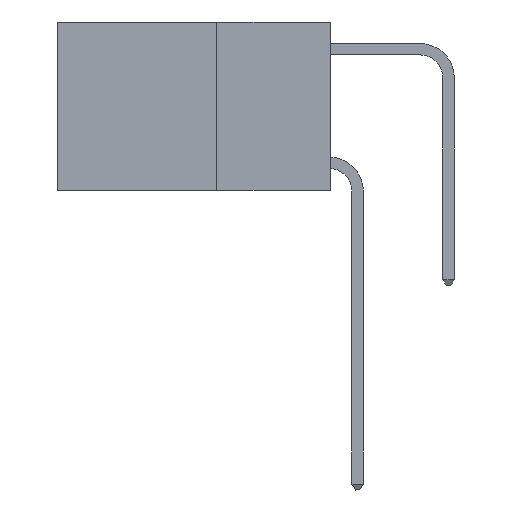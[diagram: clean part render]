
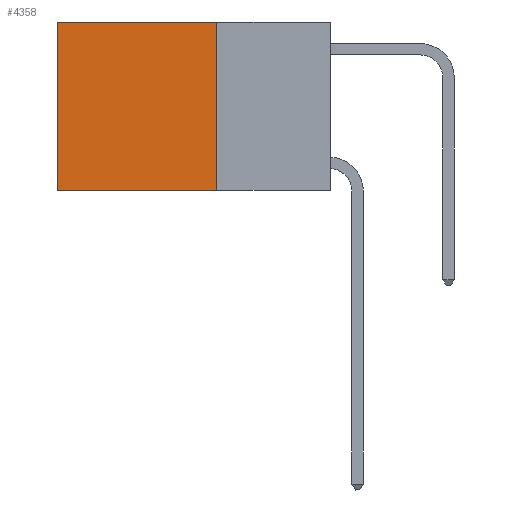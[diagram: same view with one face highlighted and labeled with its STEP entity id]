
A CAD part, left-side view. The second image highlights one B-rep face of the part: STEP entity #4358.
In plain terms, the highlighted planar face has unit normal (-1, 0, 0).
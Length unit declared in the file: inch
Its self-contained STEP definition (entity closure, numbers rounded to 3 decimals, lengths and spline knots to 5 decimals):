
#334 = EDGE_CURVE ( 'NONE', #12512, #3990, #8209, .T. ) ;
#675 = VECTOR ( 'NONE', #4784, 39.37008 ) ;
#962 = VERTEX_POINT ( 'NONE', #2156 ) ;
#1251 = EDGE_CURVE ( 'NONE', #7937, #962, #14690, .T. ) ;
#1430 = CARTESIAN_POINT ( 'NONE',  ( 0.2625, 0.25, 0. ) ) ;
#1451 = VECTOR ( 'NONE', #10331, 39.37008 ) ;
#1916 = CARTESIAN_POINT ( 'NONE',  ( 0.2625, 0.25, -0.37 ) ) ;
#2156 = CARTESIAN_POINT ( 'NONE',  ( 0.2625, 0.6, 0. ) ) ;
#3990 = VERTEX_POINT ( 'NONE', #4826 ) ;
#4358 = ADVANCED_FACE ( 'NONE', ( #16212 ), #9805, .F. ) ;
#4748 = EDGE_CURVE ( 'NONE', #7937, #12512, #12236, .T. ) ;
#4784 = DIRECTION ( 'NONE',  ( 0., 0., -1. ) ) ;
#4826 = CARTESIAN_POINT ( 'NONE',  ( 0.2625, 0.6, -0.37 ) ) ;
#5518 = DIRECTION ( 'NONE',  ( 0., 1., 0. ) ) ;
#6842 = EDGE_LOOP ( 'NONE', ( #9349, #10776, #9980, #16669 ) ) ;
#7898 = VECTOR ( 'NONE', #8095, 39.37008 ) ;
#7937 = VERTEX_POINT ( 'NONE', #1430 ) ;
#8095 = DIRECTION ( 'NONE',  ( 0., 1., 0. ) ) ;
#8209 = LINE ( 'NONE', #1916, #11579 ) ;
#8336 = AXIS2_PLACEMENT_3D ( 'NONE', #8489, #14933, #9654 ) ;
#8489 = CARTESIAN_POINT ( 'NONE',  ( 0.2625, 0.25, 0. ) ) ;
#8592 = EDGE_CURVE ( 'NONE', #962, #3990, #13028, .T. ) ;
#9349 = ORIENTED_EDGE ( 'NONE', *, *, #8592, .T. ) ;
#9654 = DIRECTION ( 'NONE',  ( 0., 0., -1. ) ) ;
#9805 = PLANE ( 'NONE',  #8336 ) ;
#9980 = ORIENTED_EDGE ( 'NONE', *, *, #4748, .F. ) ;
#10331 = DIRECTION ( 'NONE',  ( 0., 0., -1. ) ) ;
#10776 = ORIENTED_EDGE ( 'NONE', *, *, #334, .F. ) ;
#11579 = VECTOR ( 'NONE', #5518, 39.37008 ) ;
#12236 = LINE ( 'NONE', #13496, #675 ) ;
#12269 = CARTESIAN_POINT ( 'NONE',  ( 0.2625, 0.25, -0.37 ) ) ;
#12512 = VERTEX_POINT ( 'NONE', #12269 ) ;
#13028 = LINE ( 'NONE', #15395, #1451 ) ;
#13496 = CARTESIAN_POINT ( 'NONE',  ( 0.2625, 0.25, 0. ) ) ;
#14599 = CARTESIAN_POINT ( 'NONE',  ( 0.2625, 0.25, 0. ) ) ;
#14690 = LINE ( 'NONE', #14599, #7898 ) ;
#14933 = DIRECTION ( 'NONE',  ( 1., 0., 0. ) ) ;
#15395 = CARTESIAN_POINT ( 'NONE',  ( 0.2625, 0.6, 0. ) ) ;
#16212 = FACE_OUTER_BOUND ( 'NONE', #6842, .T. ) ;
#16669 = ORIENTED_EDGE ( 'NONE', *, *, #1251, .T. ) ;
